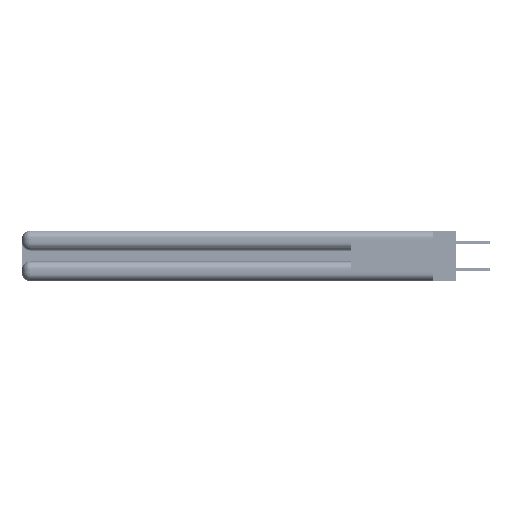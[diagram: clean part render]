
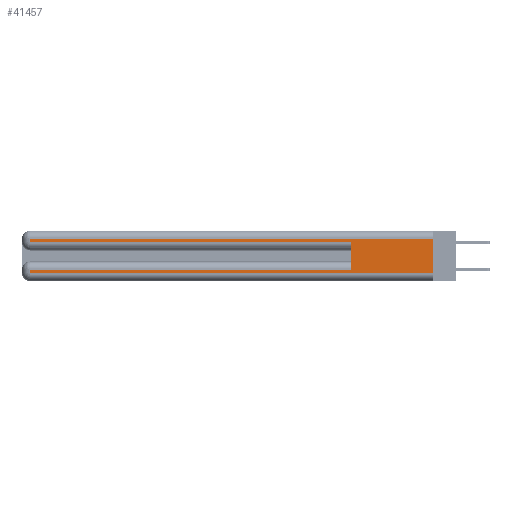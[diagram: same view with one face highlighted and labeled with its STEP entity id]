
A CAD part, left-side view. The second image highlights one B-rep face of the part: STEP entity #41457.
In plain terms, the highlighted planar face has unit normal (-1, 0, 0).
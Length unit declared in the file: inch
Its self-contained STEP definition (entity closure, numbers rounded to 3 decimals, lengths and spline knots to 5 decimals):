
#627 = VECTOR ( 'NONE', #8274, 39.37008 ) ;
#3410 = EDGE_CURVE ( 'NONE', #45574, #51736, #37098, .T. ) ;
#6124 = LINE ( 'NONE', #53310, #35075 ) ;
#6255 = DIRECTION ( 'NONE',  ( 0., -1., 0. ) ) ;
#6901 = EDGE_CURVE ( 'NONE', #51736, #22162, #52464, .T. ) ;
#6957 = CARTESIAN_POINT ( 'NONE',  ( 0., 2.94, 0.31 ) ) ;
#7712 = DIRECTION ( 'NONE',  ( 0., 0., 1. ) ) ;
#8009 = EDGE_CURVE ( 'NONE', #18193, #8714, #48047, .T. ) ;
#8274 = DIRECTION ( 'NONE',  ( 0., 0., -1. ) ) ;
#8705 = ORIENTED_EDGE ( 'NONE', *, *, #6901, .T. ) ;
#8714 = VERTEX_POINT ( 'NONE', #20358 ) ;
#9890 = DIRECTION ( 'NONE',  ( 0., 0., -1. ) ) ;
#10309 = CARTESIAN_POINT ( 'NONE',  ( 0., 0., 0.285 ) ) ;
#10532 = LINE ( 'NONE', #35005, #48057 ) ;
#12557 = DIRECTION ( 'NONE',  ( 0., -1., 0. ) ) ;
#16033 = VECTOR ( 'NONE', #12557, 39.37008 ) ;
#16061 = DIRECTION ( 'NONE',  ( 0., 1., 0. ) ) ;
#16891 = CARTESIAN_POINT ( 'NONE',  ( 0., 2.94, 0.37 ) ) ;
#18193 = VERTEX_POINT ( 'NONE', #6957 ) ;
#20358 = CARTESIAN_POINT ( 'NONE',  ( 0., 2.94, 0.285 ) ) ;
#20372 = CARTESIAN_POINT ( 'NONE',  ( 0., 0., 0.31 ) ) ;
#20849 = VERTEX_POINT ( 'NONE', #51850 ) ;
#21327 = DIRECTION ( 'NONE',  ( 0., 0., -1. ) ) ;
#22025 = CARTESIAN_POINT ( 'NONE',  ( 0., 0.6, 0.085 ) ) ;
#22162 = VERTEX_POINT ( 'NONE', #23646 ) ;
#22443 = CARTESIAN_POINT ( 'NONE',  ( 0., 0., 0.37 ) ) ;
#22673 = VECTOR ( 'NONE', #39940, 39.37008 ) ;
#23646 = CARTESIAN_POINT ( 'NONE',  ( 0., 2.94, 0.06 ) ) ;
#23957 = LINE ( 'NONE', #50063, #16033 ) ;
#25572 = CARTESIAN_POINT ( 'NONE',  ( 0., 2.94, 0.085 ) ) ;
#26316 = PLANE ( 'NONE',  #51167 ) ;
#27484 = EDGE_CURVE ( 'NONE', #22162, #32551, #23957, .T. ) ;
#27849 = VECTOR ( 'NONE', #6255, 39.37008 ) ;
#27853 = CARTESIAN_POINT ( 'NONE',  ( 0., 0., 0.06 ) ) ;
#27986 = CARTESIAN_POINT ( 'NONE',  ( 0., 0., 0.085 ) ) ;
#28071 = EDGE_CURVE ( 'NONE', #45574, #20849, #6124, .T. ) ;
#28747 = ORIENTED_EDGE ( 'NONE', *, *, #49598, .T. ) ;
#29336 = EDGE_LOOP ( 'NONE', ( #38893, #28747, #45267, #36790, #38277, #53631, #8705, #40146 ) ) ;
#32551 = VERTEX_POINT ( 'NONE', #27853 ) ;
#34412 = LINE ( 'NONE', #10309, #27849 ) ;
#35005 = CARTESIAN_POINT ( 'NONE',  ( 0., 0., 0.37 ) ) ;
#35075 = VECTOR ( 'NONE', #7712, 39.37008 ) ;
#36790 = ORIENTED_EDGE ( 'NONE', *, *, #38534, .T. ) ;
#37098 = LINE ( 'NONE', #27986, #22673 ) ;
#38277 = ORIENTED_EDGE ( 'NONE', *, *, #28071, .F. ) ;
#38534 = EDGE_CURVE ( 'NONE', #8714, #20849, #34412, .T. ) ;
#38582 = VECTOR ( 'NONE', #16061, 39.37008 ) ;
#38859 = DIRECTION ( 'NONE',  ( 0., 0., -1. ) ) ;
#38893 = ORIENTED_EDGE ( 'NONE', *, *, #46322, .F. ) ;
#39940 = DIRECTION ( 'NONE',  ( 0., 1., 0. ) ) ;
#40146 = ORIENTED_EDGE ( 'NONE', *, *, #27484, .T. ) ;
#41033 = CARTESIAN_POINT ( 'NONE',  ( 0., 2.94, 0.37 ) ) ;
#41272 = CARTESIAN_POINT ( 'NONE',  ( 0., 0., 0.31 ) ) ;
#41457 = ADVANCED_FACE ( 'NONE', ( #43331 ), #26316, .F. ) ;
#43331 = FACE_OUTER_BOUND ( 'NONE', #29336, .T. ) ;
#44483 = LINE ( 'NONE', #41272, #38582 ) ;
#45267 = ORIENTED_EDGE ( 'NONE', *, *, #8009, .T. ) ;
#45444 = VERTEX_POINT ( 'NONE', #20372 ) ;
#45574 = VERTEX_POINT ( 'NONE', #22025 ) ;
#46322 = EDGE_CURVE ( 'NONE', #45444, #32551, #10532, .T. ) ;
#46532 = VECTOR ( 'NONE', #21327, 39.37008 ) ;
#47237 = DIRECTION ( 'NONE',  ( 1., 0., 0. ) ) ;
#48047 = LINE ( 'NONE', #41033, #627 ) ;
#48057 = VECTOR ( 'NONE', #38859, 39.37008 ) ;
#49598 = EDGE_CURVE ( 'NONE', #45444, #18193, #44483, .T. ) ;
#50063 = CARTESIAN_POINT ( 'NONE',  ( 0., 0., 0.06 ) ) ;
#51167 = AXIS2_PLACEMENT_3D ( 'NONE', #22443, #47237, #9890 ) ;
#51736 = VERTEX_POINT ( 'NONE', #25572 ) ;
#51850 = CARTESIAN_POINT ( 'NONE',  ( 0., 0.6, 0.285 ) ) ;
#52464 = LINE ( 'NONE', #16891, #46532 ) ;
#53310 = CARTESIAN_POINT ( 'NONE',  ( 0., 0.6, 0.145 ) ) ;
#53631 = ORIENTED_EDGE ( 'NONE', *, *, #3410, .T. ) ;
